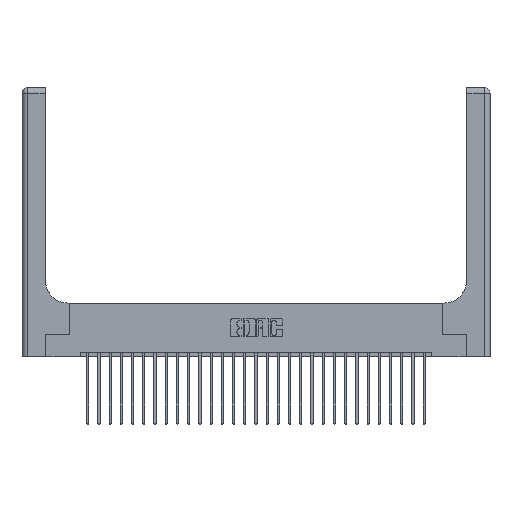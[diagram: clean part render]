
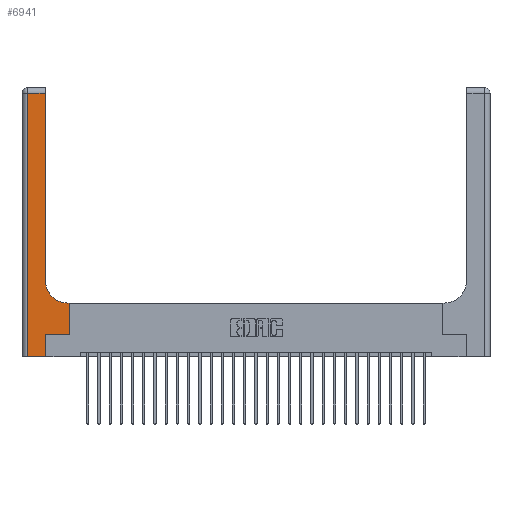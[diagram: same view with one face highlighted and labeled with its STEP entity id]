
A CAD part, top view. The second image highlights one B-rep face of the part: STEP entity #6941.
In plain terms, the highlighted planar face has unit normal (0, 0, 1).
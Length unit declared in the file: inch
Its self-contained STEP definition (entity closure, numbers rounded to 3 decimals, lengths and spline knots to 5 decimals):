
#233 = DIRECTION ( 'NONE',  ( -1., 0., 0. ) ) ;
#261 = VECTOR ( 'NONE', #10993, 39.37008 ) ;
#307 = VECTOR ( 'NONE', #10605, 39.37008 ) ;
#390 = VECTOR ( 'NONE', #9289, 39.37008 ) ;
#1679 = LINE ( 'NONE', #11936, #7182 ) ;
#1715 = CARTESIAN_POINT ( 'NONE',  ( 0.51, 0.85, 0.37 ) ) ;
#2009 = ORIENTED_EDGE ( 'NONE', *, *, #8641, .T. ) ;
#3551 = DIRECTION ( 'NONE',  ( 0., 1., 0. ) ) ;
#3750 = CARTESIAN_POINT ( 'NONE',  ( 0.26, 2.94, 0.37 ) ) ;
#4246 = EDGE_CURVE ( 'NONE', #14375, #18062, #1679, .T. ) ;
#4730 = ORIENTED_EDGE ( 'NONE', *, *, #18631, .T. ) ;
#4822 = VERTEX_POINT ( 'NONE', #11737 ) ;
#5044 = CARTESIAN_POINT ( 'NONE',  ( 0., 2.94, 0.37 ) ) ;
#5550 = ORIENTED_EDGE ( 'NONE', *, *, #11828, .T. ) ;
#5676 = CARTESIAN_POINT ( 'NONE',  ( 0.528, 0.25, 0.37 ) ) ;
#6188 = ORIENTED_EDGE ( 'NONE', *, *, #21214, .T. ) ;
#6529 = CARTESIAN_POINT ( 'NONE',  ( 0.265, 0., 0.37 ) ) ;
#6941 = ADVANCED_FACE ( 'NONE', ( #15535 ), #9249, .F. ) ;
#7182 = VECTOR ( 'NONE', #14597, 39.37008 ) ;
#7288 = LINE ( 'NONE', #25883, #25257 ) ;
#7359 = ORIENTED_EDGE ( 'NONE', *, *, #21354, .T. ) ;
#8422 = CARTESIAN_POINT ( 'NONE',  ( 0.528, 0.25, 0.37 ) ) ;
#8641 = EDGE_CURVE ( 'NONE', #19910, #4822, #13468, .T. ) ;
#8663 = DIRECTION ( 'NONE',  ( 0., 0., -1. ) ) ;
#8981 = AXIS2_PLACEMENT_3D ( 'NONE', #23864, #11381, #21859 ) ;
#9052 = ORIENTED_EDGE ( 'NONE', *, *, #16785, .T. ) ;
#9249 = PLANE ( 'NONE',  #8981 ) ;
#9289 = DIRECTION ( 'NONE',  ( 1., 0., 0. ) ) ;
#9443 = DIRECTION ( 'NONE',  ( 1., 0., 0. ) ) ;
#10605 = DIRECTION ( 'NONE',  ( 0., 1., 0. ) ) ;
#10825 = CARTESIAN_POINT ( 'NONE',  ( 0.26, 0.6, 0.37 ) ) ;
#10993 = DIRECTION ( 'NONE',  ( -1., 0., 0. ) ) ;
#11381 = DIRECTION ( 'NONE',  ( 0., 0., -1. ) ) ;
#11395 = EDGE_LOOP ( 'NONE', ( #6188, #7359, #4730, #22207, #25942, #23824, #9052, #2009, #5550 ) ) ;
#11737 = CARTESIAN_POINT ( 'NONE',  ( 0.51, 0.6, 0.37 ) ) ;
#11828 = EDGE_CURVE ( 'NONE', #4822, #26307, #26324, .T. ) ;
#11936 = CARTESIAN_POINT ( 'NONE',  ( 0.265, 0., 0.37 ) ) ;
#12734 = CARTESIAN_POINT ( 'NONE',  ( 0.06, 0., 0.37 ) ) ;
#12791 = CARTESIAN_POINT ( 'NONE',  ( 0.265, 0.25, 0.37 ) ) ;
#13468 = LINE ( 'NONE', #10825, #21932 ) ;
#13784 = CARTESIAN_POINT ( 'NONE',  ( 0.265, 0.25, 0.37 ) ) ;
#14375 = VERTEX_POINT ( 'NONE', #6529 ) ;
#14597 = DIRECTION ( 'NONE',  ( 0., 1., 0. ) ) ;
#14955 = LINE ( 'NONE', #8422, #307 ) ;
#15183 = VECTOR ( 'NONE', #24601, 39.37008 ) ;
#15535 = FACE_OUTER_BOUND ( 'NONE', #11395, .T. ) ;
#15616 = CARTESIAN_POINT ( 'NONE',  ( 0., 0., 0.37 ) ) ;
#16323 = CARTESIAN_POINT ( 'NONE',  ( 0.26, 3., 0.37 ) ) ;
#16785 = EDGE_CURVE ( 'NONE', #20860, #19910, #14955, .T. ) ;
#17257 = DIRECTION ( 'NONE',  ( 0., -1., 0. ) ) ;
#17310 = VERTEX_POINT ( 'NONE', #12734 ) ;
#17574 = CARTESIAN_POINT ( 'NONE',  ( 0.06, 2.94, 0.37 ) ) ;
#17637 = LINE ( 'NONE', #15616, #390 ) ;
#18062 = VERTEX_POINT ( 'NONE', #12791 ) ;
#18326 = EDGE_CURVE ( 'NONE', #18062, #20860, #21383, .T. ) ;
#18415 = VERTEX_POINT ( 'NONE', #3750 ) ;
#18631 = EDGE_CURVE ( 'NONE', #21459, #17310, #7288, .T. ) ;
#19910 = VERTEX_POINT ( 'NONE', #21471 ) ;
#20236 = LINE ( 'NONE', #16323, #26755 ) ;
#20860 = VERTEX_POINT ( 'NONE', #5676 ) ;
#21214 = EDGE_CURVE ( 'NONE', #26307, #18415, #20236, .T. ) ;
#21354 = EDGE_CURVE ( 'NONE', #18415, #21459, #22090, .T. ) ;
#21383 = LINE ( 'NONE', #13784, #15183 ) ;
#21459 = VERTEX_POINT ( 'NONE', #17574 ) ;
#21471 = CARTESIAN_POINT ( 'NONE',  ( 0.528, 0.6, 0.37 ) ) ;
#21803 = EDGE_CURVE ( 'NONE', #17310, #14375, #17637, .T. ) ;
#21859 = DIRECTION ( 'NONE',  ( -1., 0., 0. ) ) ;
#21932 = VECTOR ( 'NONE', #233, 39.37008 ) ;
#22090 = LINE ( 'NONE', #5044, #261 ) ;
#22207 = ORIENTED_EDGE ( 'NONE', *, *, #21803, .T. ) ;
#23824 = ORIENTED_EDGE ( 'NONE', *, *, #18326, .T. ) ;
#23864 = CARTESIAN_POINT ( 'NONE',  ( 0., 3., 0.37 ) ) ;
#24601 = DIRECTION ( 'NONE',  ( 1., 0., 0. ) ) ;
#24965 = AXIS2_PLACEMENT_3D ( 'NONE', #1715, #8663, #9443 ) ;
#25257 = VECTOR ( 'NONE', #17257, 39.37008 ) ;
#25742 = CARTESIAN_POINT ( 'NONE',  ( 0.26, 0.85, 0.37 ) ) ;
#25883 = CARTESIAN_POINT ( 'NONE',  ( 0.06, 3., 0.37 ) ) ;
#25942 = ORIENTED_EDGE ( 'NONE', *, *, #4246, .T. ) ;
#26307 = VERTEX_POINT ( 'NONE', #25742 ) ;
#26324 = CIRCLE ( 'NONE', #24965, 0.25 ) ;
#26755 = VECTOR ( 'NONE', #3551, 39.37008 ) ;
